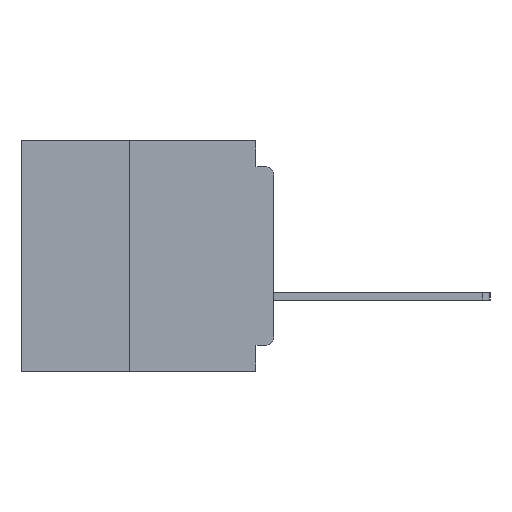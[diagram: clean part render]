
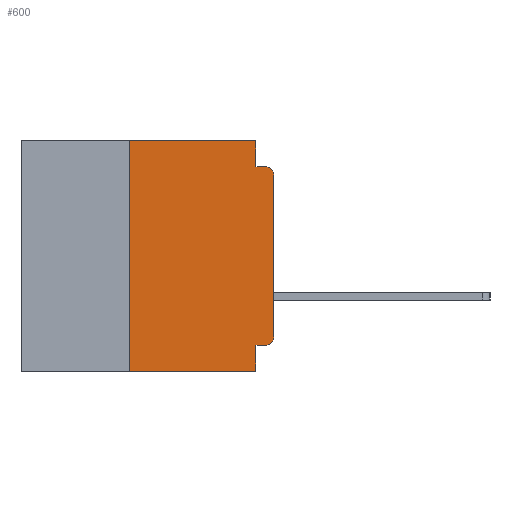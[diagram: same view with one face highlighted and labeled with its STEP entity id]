
A CAD part, left-side view. The second image highlights one B-rep face of the part: STEP entity #600.
In plain terms, the highlighted planar face has unit normal (-1, 0, 0).
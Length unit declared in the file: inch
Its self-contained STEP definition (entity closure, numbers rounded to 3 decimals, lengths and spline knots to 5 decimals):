
#423 = DIRECTION ( 'NONE',  ( 0., 0., 1. ) ) ;
#600 = ADVANCED_FACE ( 'NONE', ( #14959 ), #34549, .F. ) ;
#1987 = EDGE_CURVE ( 'NONE', #40117, #17797, #11567, .T. ) ;
#2553 = LINE ( 'NONE', #10548, #35082 ) ;
#3805 = CARTESIAN_POINT ( 'NONE',  ( 0., 0.25, 0. ) ) ;
#3851 = CARTESIAN_POINT ( 'NONE',  ( 0., 0.437, 0. ) ) ;
#5752 = VERTEX_POINT ( 'NONE', #3805 ) ;
#6515 = CARTESIAN_POINT ( 'NONE',  ( 0., 0., -0.34 ) ) ;
#6523 = ORIENTED_EDGE ( 'NONE', *, *, #31303, .F. ) ;
#6921 = LINE ( 'NONE', #3851, #27771 ) ;
#7165 = ORIENTED_EDGE ( 'NONE', *, *, #9042, .T. ) ;
#7332 = EDGE_CURVE ( 'NONE', #49910, #17797, #46000, .T. ) ;
#7438 = EDGE_CURVE ( 'NONE', #50896, #7727, #40798, .T. ) ;
#7727 = VERTEX_POINT ( 'NONE', #31584 ) ;
#7890 = CIRCLE ( 'NONE', #46060, 0.015 ) ;
#8106 = DIRECTION ( 'NONE',  ( 0., -1., 0. ) ) ;
#8383 = LINE ( 'NONE', #8801, #29159 ) ;
#8546 = ORIENTED_EDGE ( 'NONE', *, *, #50222, .T. ) ;
#8801 = CARTESIAN_POINT ( 'NONE',  ( 0., 0., -0.355 ) ) ;
#8842 = CARTESIAN_POINT ( 'NONE',  ( 0., 0.031, -0.4 ) ) ;
#9042 = EDGE_CURVE ( 'NONE', #10535, #7727, #30291, .T. ) ;
#9322 = AXIS2_PLACEMENT_3D ( 'NONE', #34922, #34480, #34383 ) ;
#9986 = DIRECTION ( 'NONE',  ( 0., 0., -1. ) ) ;
#10535 = VERTEX_POINT ( 'NONE', #34167 ) ;
#10548 = CARTESIAN_POINT ( 'NONE',  ( 0., 0.25, -0.4 ) ) ;
#10817 = VECTOR ( 'NONE', #24034, 39.37008 ) ;
#11458 = CARTESIAN_POINT ( 'NONE',  ( 0., 0.031, 0. ) ) ;
#11475 = CARTESIAN_POINT ( 'NONE',  ( 0., 0.015, -0.06 ) ) ;
#11567 = LINE ( 'NONE', #8842, #34747 ) ;
#11974 = DIRECTION ( 'NONE',  ( -1., 0., 0. ) ) ;
#12523 = CARTESIAN_POINT ( 'NONE',  ( 0., 0.437, -0.4 ) ) ;
#13065 = DIRECTION ( 'NONE',  ( 0., 1., 0. ) ) ;
#14959 = FACE_OUTER_BOUND ( 'NONE', #20832, .T. ) ;
#15738 = DIRECTION ( 'NONE',  ( 0., 0., -1. ) ) ;
#15853 = VERTEX_POINT ( 'NONE', #34070 ) ;
#17797 = VERTEX_POINT ( 'NONE', #46112 ) ;
#18973 = VECTOR ( 'NONE', #25768, 39.37008 ) ;
#20151 = LINE ( 'NONE', #33645, #49017 ) ;
#20832 = EDGE_LOOP ( 'NONE', ( #27997, #7165, #23544, #45384, #38228, #6523, #42172, #46072, #29316, #8546 ) ) ;
#21810 = EDGE_CURVE ( 'NONE', #35369, #10535, #20151, .T. ) ;
#22234 = CARTESIAN_POINT ( 'NONE',  ( 0., 0.25, -0.4 ) ) ;
#23544 = ORIENTED_EDGE ( 'NONE', *, *, #7438, .F. ) ;
#24034 = DIRECTION ( 'NONE',  ( 0., 0., -1. ) ) ;
#25768 = DIRECTION ( 'NONE',  ( 0., -1., 0. ) ) ;
#27771 = VECTOR ( 'NONE', #8106, 39.37008 ) ;
#27915 = AXIS2_PLACEMENT_3D ( 'NONE', #11475, #40337, #15738 ) ;
#27997 = ORIENTED_EDGE ( 'NONE', *, *, #21810, .T. ) ;
#29159 = VECTOR ( 'NONE', #13065, 39.37008 ) ;
#29316 = ORIENTED_EDGE ( 'NONE', *, *, #52247, .F. ) ;
#29839 = CARTESIAN_POINT ( 'NONE',  ( 0., 0., -0.045 ) ) ;
#30291 = CIRCLE ( 'NONE', #27915, 0.015 ) ;
#31303 = EDGE_CURVE ( 'NONE', #49910, #5752, #2553, .T. ) ;
#31584 = CARTESIAN_POINT ( 'NONE',  ( 0., 0.015, -0.045 ) ) ;
#33645 = CARTESIAN_POINT ( 'NONE',  ( 0., 0., 0. ) ) ;
#34070 = CARTESIAN_POINT ( 'NONE',  ( 0., 0.031, 0. ) ) ;
#34167 = CARTESIAN_POINT ( 'NONE',  ( 0., 0., -0.06 ) ) ;
#34383 = DIRECTION ( 'NONE',  ( 0., 0., -1. ) ) ;
#34480 = DIRECTION ( 'NONE',  ( 1., 0., 0. ) ) ;
#34549 = PLANE ( 'NONE',  #9322 ) ;
#34747 = VECTOR ( 'NONE', #9986, 39.37008 ) ;
#34922 = CARTESIAN_POINT ( 'NONE',  ( 0., 0.437, 0. ) ) ;
#34943 = VECTOR ( 'NONE', #37167, 39.37008 ) ;
#35082 = VECTOR ( 'NONE', #47576, 39.37008 ) ;
#35369 = VERTEX_POINT ( 'NONE', #6515 ) ;
#35577 = VERTEX_POINT ( 'NONE', #36876 ) ;
#36107 = EDGE_CURVE ( 'NONE', #5752, #15853, #6921, .T. ) ;
#36643 = CARTESIAN_POINT ( 'NONE',  ( 0., 0.015, -0.34 ) ) ;
#36876 = CARTESIAN_POINT ( 'NONE',  ( 0., 0.015, -0.355 ) ) ;
#37167 = DIRECTION ( 'NONE',  ( 0., -1., 0. ) ) ;
#38228 = ORIENTED_EDGE ( 'NONE', *, *, #36107, .F. ) ;
#40117 = VERTEX_POINT ( 'NONE', #51946 ) ;
#40337 = DIRECTION ( 'NONE',  ( -1., 0., 0. ) ) ;
#40798 = LINE ( 'NONE', #29839, #18973 ) ;
#40844 = DIRECTION ( 'NONE',  ( 0., 0., -1. ) ) ;
#42172 = ORIENTED_EDGE ( 'NONE', *, *, #7332, .T. ) ;
#45066 = LINE ( 'NONE', #11458, #10817 ) ;
#45384 = ORIENTED_EDGE ( 'NONE', *, *, #46758, .F. ) ;
#46000 = LINE ( 'NONE', #12523, #34943 ) ;
#46060 = AXIS2_PLACEMENT_3D ( 'NONE', #36643, #11974, #40844 ) ;
#46072 = ORIENTED_EDGE ( 'NONE', *, *, #1987, .F. ) ;
#46112 = CARTESIAN_POINT ( 'NONE',  ( 0., 0.031, -0.4 ) ) ;
#46758 = EDGE_CURVE ( 'NONE', #15853, #50896, #45066, .T. ) ;
#47576 = DIRECTION ( 'NONE',  ( 0., 0., 1. ) ) ;
#49017 = VECTOR ( 'NONE', #423, 39.37008 ) ;
#49391 = CARTESIAN_POINT ( 'NONE',  ( 0., 0.031, -0.045 ) ) ;
#49910 = VERTEX_POINT ( 'NONE', #22234 ) ;
#50222 = EDGE_CURVE ( 'NONE', #35577, #35369, #7890, .T. ) ;
#50896 = VERTEX_POINT ( 'NONE', #49391 ) ;
#51946 = CARTESIAN_POINT ( 'NONE',  ( 0., 0.031, -0.355 ) ) ;
#52247 = EDGE_CURVE ( 'NONE', #35577, #40117, #8383, .T. ) ;
